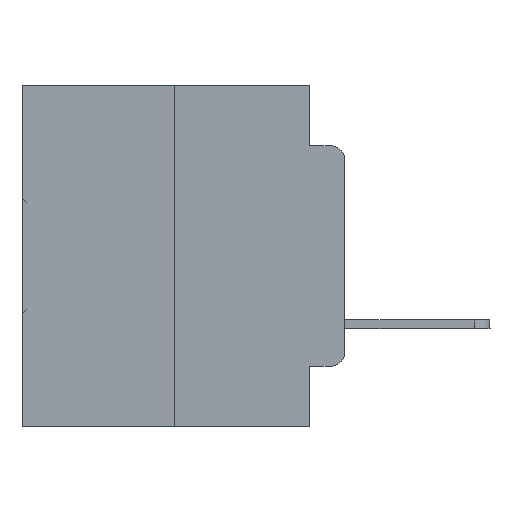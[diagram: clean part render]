
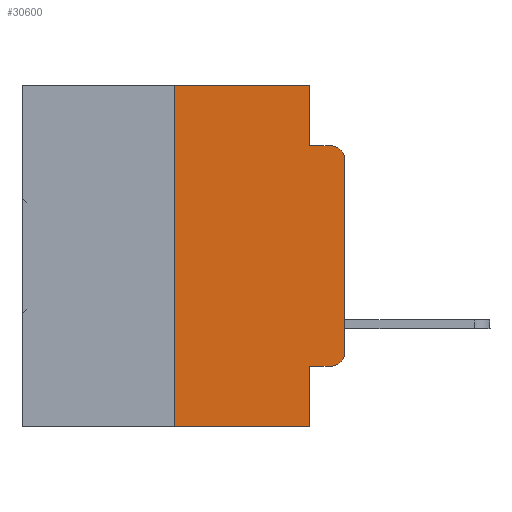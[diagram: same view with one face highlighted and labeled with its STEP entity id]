
A CAD part, left-side view. The second image highlights one B-rep face of the part: STEP entity #30600.
In plain terms, the highlighted planar face has unit normal (-1, 0, 0).
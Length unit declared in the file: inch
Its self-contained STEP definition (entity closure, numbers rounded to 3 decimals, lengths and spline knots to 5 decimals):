
#1047 = VERTEX_POINT ( 'NONE', #4444 ) ;
#1061 = LINE ( 'NONE', #8370, #29997 ) ;
#1128 = VERTEX_POINT ( 'NONE', #12540 ) ;
#1547 = CARTESIAN_POINT ( 'NONE',  ( 0., 0.051, 0. ) ) ;
#1991 = CARTESIAN_POINT ( 'NONE',  ( 0., 0.051, -0.5 ) ) ;
#2041 = ORIENTED_EDGE ( 'NONE', *, *, #20693, .T. ) ;
#2461 = EDGE_CURVE ( 'NONE', #6115, #1128, #6454, .T. ) ;
#2750 = LINE ( 'NONE', #3719, #10906 ) ;
#3280 = DIRECTION ( 'NONE',  ( 0., 0., 1. ) ) ;
#3319 = ORIENTED_EDGE ( 'NONE', *, *, #17016, .T. ) ;
#3338 = VECTOR ( 'NONE', #18889, 39.37008 ) ;
#3719 = CARTESIAN_POINT ( 'NONE',  ( 0., 0.473, 0. ) ) ;
#4444 = CARTESIAN_POINT ( 'NONE',  ( 0., 0., -0.3915 ) ) ;
#5172 = CARTESIAN_POINT ( 'NONE',  ( 0., 0.25, -0.5 ) ) ;
#5542 = CARTESIAN_POINT ( 'NONE',  ( 0., 0.25, 0. ) ) ;
#5709 = EDGE_CURVE ( 'NONE', #7188, #20234, #1061, .T. ) ;
#6115 = VERTEX_POINT ( 'NONE', #28611 ) ;
#6292 = DIRECTION ( 'NONE',  ( 0., 0., -1. ) ) ;
#6381 = VECTOR ( 'NONE', #8091, 39.37008 ) ;
#6435 = CARTESIAN_POINT ( 'NONE',  ( 0., 0.02, -0.4115 ) ) ;
#6454 = LINE ( 'NONE', #6496, #3338 ) ;
#6496 = CARTESIAN_POINT ( 'NONE',  ( 0., 0.051, -0.0885 ) ) ;
#7188 = VERTEX_POINT ( 'NONE', #31514 ) ;
#7735 = DIRECTION ( 'NONE',  ( 0., -1., 0. ) ) ;
#8036 = FACE_OUTER_BOUND ( 'NONE', #26297, .T. ) ;
#8091 = DIRECTION ( 'NONE',  ( 0., 0., 1. ) ) ;
#8197 = ORIENTED_EDGE ( 'NONE', *, *, #2461, .F. ) ;
#8370 = CARTESIAN_POINT ( 'NONE',  ( 0., 0.051, -0.4115 ) ) ;
#8853 = LINE ( 'NONE', #22486, #26887 ) ;
#9305 = EDGE_CURVE ( 'NONE', #12308, #1128, #24800, .T. ) ;
#9584 = CARTESIAN_POINT ( 'NONE',  ( 0., 0.02, -0.3915 ) ) ;
#9682 = DIRECTION ( 'NONE',  ( 0., 0., -1. ) ) ;
#9916 = EDGE_CURVE ( 'NONE', #30316, #30549, #29371, .T. ) ;
#10107 = LINE ( 'NONE', #18153, #15091 ) ;
#10906 = VECTOR ( 'NONE', #31213, 39.37008 ) ;
#11081 = DIRECTION ( 'NONE',  ( 0., 0., -1. ) ) ;
#11159 = ORIENTED_EDGE ( 'NONE', *, *, #13486, .F. ) ;
#11290 = VERTEX_POINT ( 'NONE', #1991 ) ;
#12308 = VERTEX_POINT ( 'NONE', #17207 ) ;
#12540 = CARTESIAN_POINT ( 'NONE',  ( 0., 0.02, -0.0885 ) ) ;
#13020 = EDGE_CURVE ( 'NONE', #30549, #31243, #2750, .T. ) ;
#13486 = EDGE_CURVE ( 'NONE', #7188, #11290, #10107, .T. ) ;
#15091 = VECTOR ( 'NONE', #18270, 39.37008 ) ;
#15835 = CARTESIAN_POINT ( 'NONE',  ( 0., 0.02, -0.1085 ) ) ;
#17016 = EDGE_CURVE ( 'NONE', #30316, #11290, #8853, .T. ) ;
#17207 = CARTESIAN_POINT ( 'NONE',  ( 0., 0., -0.1085 ) ) ;
#18153 = CARTESIAN_POINT ( 'NONE',  ( 0., 0.051, 0. ) ) ;
#18270 = DIRECTION ( 'NONE',  ( 0., 0., -1. ) ) ;
#18800 = ORIENTED_EDGE ( 'NONE', *, *, #5709, .T. ) ;
#18889 = DIRECTION ( 'NONE',  ( 0., -1., 0. ) ) ;
#19499 = ORIENTED_EDGE ( 'NONE', *, *, #25947, .F. ) ;
#20234 = VERTEX_POINT ( 'NONE', #6435 ) ;
#20479 = CARTESIAN_POINT ( 'NONE',  ( 0., 0.25, 0. ) ) ;
#20565 = CARTESIAN_POINT ( 'NONE',  ( 0., 0., 0. ) ) ;
#20628 = LINE ( 'NONE', #20565, #6381 ) ;
#20693 = EDGE_CURVE ( 'NONE', #20234, #1047, #24522, .T. ) ;
#20986 = EDGE_CURVE ( 'NONE', #1047, #12308, #20628, .T. ) ;
#21039 = CARTESIAN_POINT ( 'NONE',  ( 0., 0.473, 0. ) ) ;
#21134 = ORIENTED_EDGE ( 'NONE', *, *, #9916, .F. ) ;
#22248 = AXIS2_PLACEMENT_3D ( 'NONE', #15835, #30782, #11081 ) ;
#22486 = CARTESIAN_POINT ( 'NONE',  ( 0., 0.473, -0.5 ) ) ;
#23091 = AXIS2_PLACEMENT_3D ( 'NONE', #21039, #23521, #23630 ) ;
#23449 = ORIENTED_EDGE ( 'NONE', *, *, #13020, .F. ) ;
#23521 = DIRECTION ( 'NONE',  ( 1., 0., 0. ) ) ;
#23630 = DIRECTION ( 'NONE',  ( 0., 0., -1. ) ) ;
#24522 = CIRCLE ( 'NONE', #28482, 0.02 ) ;
#24800 = CIRCLE ( 'NONE', #22248, 0.02 ) ;
#25906 = DIRECTION ( 'NONE',  ( 0., -1., 0. ) ) ;
#25947 = EDGE_CURVE ( 'NONE', #31243, #6115, #28363, .T. ) ;
#26297 = EDGE_LOOP ( 'NONE', ( #26674, #28018, #8197, #19499, #23449, #21134, #3319, #11159, #18800, #2041 ) ) ;
#26674 = ORIENTED_EDGE ( 'NONE', *, *, #20986, .T. ) ;
#26758 = DIRECTION ( 'NONE',  ( -1., 0., 0. ) ) ;
#26887 = VECTOR ( 'NONE', #7735, 39.37008 ) ;
#28018 = ORIENTED_EDGE ( 'NONE', *, *, #9305, .T. ) ;
#28363 = LINE ( 'NONE', #1547, #29904 ) ;
#28482 = AXIS2_PLACEMENT_3D ( 'NONE', #9584, #26758, #9682 ) ;
#28555 = CARTESIAN_POINT ( 'NONE',  ( 0., 0.051, 0. ) ) ;
#28611 = CARTESIAN_POINT ( 'NONE',  ( 0., 0.051, -0.0885 ) ) ;
#29371 = LINE ( 'NONE', #5542, #31706 ) ;
#29904 = VECTOR ( 'NONE', #6292, 39.37008 ) ;
#29997 = VECTOR ( 'NONE', #25906, 39.37008 ) ;
#30316 = VERTEX_POINT ( 'NONE', #5172 ) ;
#30549 = VERTEX_POINT ( 'NONE', #20479 ) ;
#30600 = ADVANCED_FACE ( 'NONE', ( #8036 ), #30939, .F. ) ;
#30782 = DIRECTION ( 'NONE',  ( -1., 0., 0. ) ) ;
#30939 = PLANE ( 'NONE',  #23091 ) ;
#31213 = DIRECTION ( 'NONE',  ( 0., -1., 0. ) ) ;
#31243 = VERTEX_POINT ( 'NONE', #28555 ) ;
#31514 = CARTESIAN_POINT ( 'NONE',  ( 0., 0.051, -0.4115 ) ) ;
#31706 = VECTOR ( 'NONE', #3280, 39.37008 ) ;
